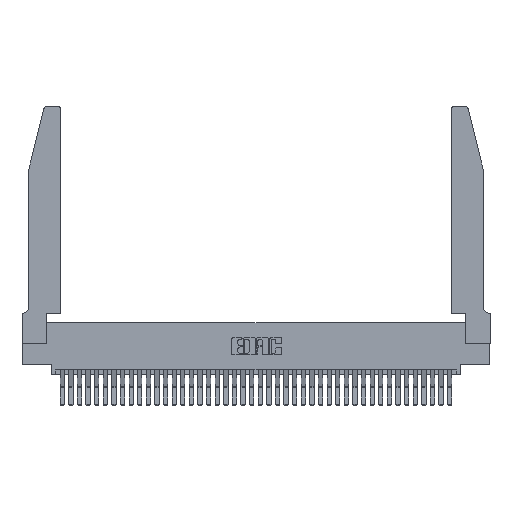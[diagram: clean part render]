
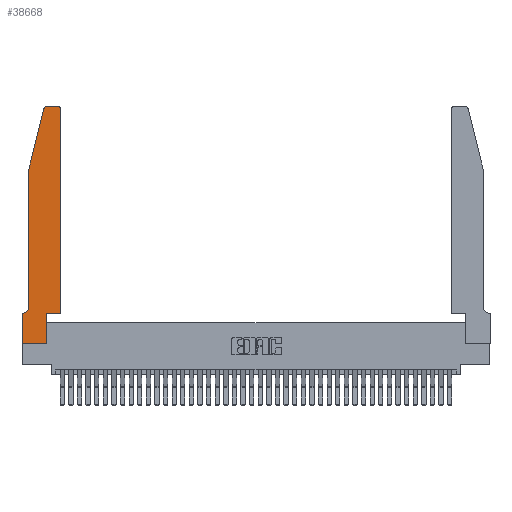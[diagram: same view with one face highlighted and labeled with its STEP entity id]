
A CAD part, top view. The second image highlights one B-rep face of the part: STEP entity #38668.
In plain terms, the highlighted planar face has unit normal (0, 0, 1).
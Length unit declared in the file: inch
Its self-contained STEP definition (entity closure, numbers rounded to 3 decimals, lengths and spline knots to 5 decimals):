
#40 = EDGE_CURVE ( 'NONE', #36649, #2752, #30031, .T. ) ;
#120 = ORIENTED_EDGE ( 'NONE', *, *, #21947, .T. ) ;
#162 = LINE ( 'NONE', #32671, #21761 ) ;
#356 = EDGE_CURVE ( 'NONE', #35258, #21524, #162, .T. ) ;
#678 = VERTEX_POINT ( 'NONE', #22990 ) ;
#1846 = ORIENTED_EDGE ( 'NONE', *, *, #22365, .T. ) ;
#2022 = VECTOR ( 'NONE', #22735, 39.37008 ) ;
#2062 = CIRCLE ( 'NONE', #19074, 0.03 ) ;
#2088 = EDGE_LOOP ( 'NONE', ( #16582, #120, #27021, #40327, #36115, #37939, #1846, #9252, #38995, #17040, #38059, #7077 ) ) ;
#2127 = VECTOR ( 'NONE', #17399, 39.37008 ) ;
#2670 = CARTESIAN_POINT ( 'NONE',  ( 0., 0., 0.37 ) ) ;
#2752 = VERTEX_POINT ( 'NONE', #21137 ) ;
#3942 = CARTESIAN_POINT ( 'NONE',  ( 0.25487, 2.72718, 0.37 ) ) ;
#4390 = CARTESIAN_POINT ( 'NONE',  ( 0.4205, 2.72, 0.37 ) ) ;
#5508 = CARTESIAN_POINT ( 'NONE',  ( 0.2865, 0.35, 0.37 ) ) ;
#5944 = EDGE_CURVE ( 'NONE', #35034, #36649, #37931, .T. ) ;
#6235 = EDGE_CURVE ( 'NONE', #21524, #18022, #19766, .T. ) ;
#6404 = EDGE_CURVE ( 'NONE', #18022, #35034, #25152, .T. ) ;
#6791 = CARTESIAN_POINT ( 'NONE',  ( 0.4505, 2.72, 0.37 ) ) ;
#7077 = ORIENTED_EDGE ( 'NONE', *, *, #40, .T. ) ;
#7151 = CARTESIAN_POINT ( 'NONE',  ( 0.0755, 0.42, 0.37 ) ) ;
#8014 = DIRECTION ( 'NONE',  ( 1., 0., 0. ) ) ;
#8478 = CARTESIAN_POINT ( 'NONE',  ( 0.4505, 0.35, 0.37 ) ) ;
#9166 = DIRECTION ( 'NONE',  ( 0., 1., 0. ) ) ;
#9252 = ORIENTED_EDGE ( 'NONE', *, *, #356, .T. ) ;
#9508 = CARTESIAN_POINT ( 'NONE',  ( 0.0055, 0.35, 0.37 ) ) ;
#10008 = DIRECTION ( 'NONE',  ( -0.239, -0.971, 0. ) ) ;
#10337 = LINE ( 'NONE', #13808, #2022 ) ;
#10853 = CARTESIAN_POINT ( 'NONE',  ( 0.284, 2.72, 0.37 ) ) ;
#10927 = DIRECTION ( 'NONE',  ( 0., 0., 1. ) ) ;
#13808 = CARTESIAN_POINT ( 'NONE',  ( 0., 0., 0.37 ) ) ;
#15088 = CIRCLE ( 'NONE', #15582, 0.07 ) ;
#15107 = VERTEX_POINT ( 'NONE', #7151 ) ;
#15582 = AXIS2_PLACEMENT_3D ( 'NONE', #26273, #32823, #23423 ) ;
#16582 = ORIENTED_EDGE ( 'NONE', *, *, #17096, .T. ) ;
#16704 = LINE ( 'NONE', #21449, #25488 ) ;
#16944 = VERTEX_POINT ( 'NONE', #3942 ) ;
#17040 = ORIENTED_EDGE ( 'NONE', *, *, #6404, .T. ) ;
#17096 = EDGE_CURVE ( 'NONE', #2752, #678, #36755, .T. ) ;
#17399 = DIRECTION ( 'NONE',  ( 0., 1., 0. ) ) ;
#18022 = VERTEX_POINT ( 'NONE', #5508 ) ;
#18754 = CARTESIAN_POINT ( 'NONE',  ( 0.2865, 0.35, 0.37 ) ) ;
#19036 = EDGE_CURVE ( 'NONE', #15107, #21746, #15088, .T. ) ;
#19074 = AXIS2_PLACEMENT_3D ( 'NONE', #10853, #32906, #23501 ) ;
#19642 = CARTESIAN_POINT ( 'NONE',  ( 0.0755, 2., 0.37 ) ) ;
#19766 = LINE ( 'NONE', #18754, #35445 ) ;
#20487 = CARTESIAN_POINT ( 'NONE',  ( 0., 0.35, 0.37 ) ) ;
#21088 = DIRECTION ( 'NONE',  ( 0., 0., 1. ) ) ;
#21137 = CARTESIAN_POINT ( 'NONE',  ( 0.4205, 2.75, 0.37 ) ) ;
#21449 = CARTESIAN_POINT ( 'NONE',  ( 0.0755, 0.35, 0.37 ) ) ;
#21524 = VERTEX_POINT ( 'NONE', #37332 ) ;
#21746 = VERTEX_POINT ( 'NONE', #9508 ) ;
#21761 = VECTOR ( 'NONE', #39275, 39.37008 ) ;
#21947 = EDGE_CURVE ( 'NONE', #678, #16944, #2062, .T. ) ;
#22365 = EDGE_CURVE ( 'NONE', #26577, #35258, #10337, .T. ) ;
#22735 = DIRECTION ( 'NONE',  ( 0., -1., 0. ) ) ;
#22990 = CARTESIAN_POINT ( 'NONE',  ( 0.284, 2.75, 0.37 ) ) ;
#23423 = DIRECTION ( 'NONE',  ( -1., 0., 0. ) ) ;
#23501 = DIRECTION ( 'NONE',  ( 1., 0., 0. ) ) ;
#24086 = DIRECTION ( 'NONE',  ( 1., 0., 0. ) ) ;
#25152 = LINE ( 'NONE', #27420, #25647 ) ;
#25488 = VECTOR ( 'NONE', #27861, 39.37008 ) ;
#25647 = VECTOR ( 'NONE', #40155, 39.37008 ) ;
#25790 = LINE ( 'NONE', #19642, #40026 ) ;
#26273 = CARTESIAN_POINT ( 'NONE',  ( 0.0055, 0.42, 0.37 ) ) ;
#26577 = VERTEX_POINT ( 'NONE', #20487 ) ;
#27021 = ORIENTED_EDGE ( 'NONE', *, *, #27120, .T. ) ;
#27120 = EDGE_CURVE ( 'NONE', #16944, #40150, #25790, .T. ) ;
#27420 = CARTESIAN_POINT ( 'NONE',  ( 0.4505, 0.35, 0.37 ) ) ;
#27861 = DIRECTION ( 'NONE',  ( -1., 0., 0. ) ) ;
#28194 = VECTOR ( 'NONE', #34635, 39.37008 ) ;
#28892 = VECTOR ( 'NONE', #33203, 39.37008 ) ;
#30031 = CIRCLE ( 'NONE', #31373, 0.03 ) ;
#30141 = LINE ( 'NONE', #31872, #28194 ) ;
#31373 = AXIS2_PLACEMENT_3D ( 'NONE', #4390, #10927, #8014 ) ;
#31872 = CARTESIAN_POINT ( 'NONE',  ( 0.0755, 2., 0.37 ) ) ;
#32457 = EDGE_CURVE ( 'NONE', #40150, #15107, #30141, .T. ) ;
#32577 = AXIS2_PLACEMENT_3D ( 'NONE', #36840, #21088, #24086 ) ;
#32671 = CARTESIAN_POINT ( 'NONE',  ( 0., 0., 0.37 ) ) ;
#32823 = DIRECTION ( 'NONE',  ( 0., 0., -1. ) ) ;
#32906 = DIRECTION ( 'NONE',  ( 0., 0., 1. ) ) ;
#33203 = DIRECTION ( 'NONE',  ( -1., 0., 0. ) ) ;
#34635 = DIRECTION ( 'NONE',  ( 0., -1., 0. ) ) ;
#35034 = VERTEX_POINT ( 'NONE', #39665 ) ;
#35258 = VERTEX_POINT ( 'NONE', #2670 ) ;
#35445 = VECTOR ( 'NONE', #9166, 39.37008 ) ;
#35856 = EDGE_CURVE ( 'NONE', #21746, #26577, #16704, .T. ) ;
#36115 = ORIENTED_EDGE ( 'NONE', *, *, #19036, .T. ) ;
#36239 = CARTESIAN_POINT ( 'NONE',  ( 0.2605, 2.75, 0.37 ) ) ;
#36649 = VERTEX_POINT ( 'NONE', #6791 ) ;
#36755 = LINE ( 'NONE', #36239, #28892 ) ;
#36840 = CARTESIAN_POINT ( 'NONE',  ( 0., 0.35, 0.37 ) ) ;
#37332 = CARTESIAN_POINT ( 'NONE',  ( 0.2865, 0., 0.37 ) ) ;
#37931 = LINE ( 'NONE', #8478, #2127 ) ;
#37939 = ORIENTED_EDGE ( 'NONE', *, *, #35856, .T. ) ;
#38019 = FACE_OUTER_BOUND ( 'NONE', #2088, .T. ) ;
#38059 = ORIENTED_EDGE ( 'NONE', *, *, #5944, .T. ) ;
#38668 = ADVANCED_FACE ( 'NONE', ( #38019 ), #39416, .T. ) ;
#38995 = ORIENTED_EDGE ( 'NONE', *, *, #6235, .T. ) ;
#39275 = DIRECTION ( 'NONE',  ( 1., 0., 0. ) ) ;
#39416 = PLANE ( 'NONE',  #32577 ) ;
#39665 = CARTESIAN_POINT ( 'NONE',  ( 0.4505, 0.35, 0.37 ) ) ;
#39726 = CARTESIAN_POINT ( 'NONE',  ( 0.0755, 2., 0.37 ) ) ;
#40026 = VECTOR ( 'NONE', #10008, 39.37008 ) ;
#40150 = VERTEX_POINT ( 'NONE', #39726 ) ;
#40155 = DIRECTION ( 'NONE',  ( 1., 0., 0. ) ) ;
#40327 = ORIENTED_EDGE ( 'NONE', *, *, #32457, .T. ) ;
